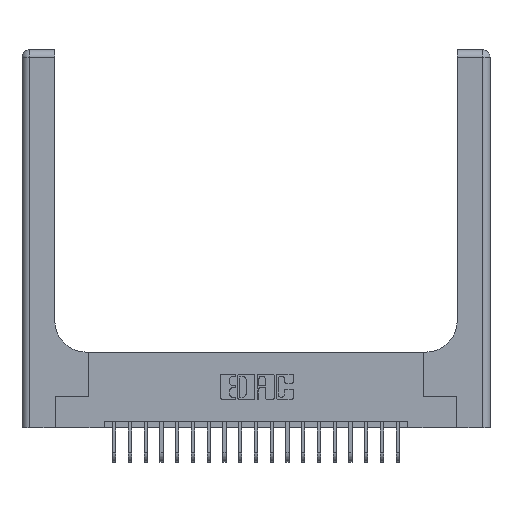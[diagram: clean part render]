
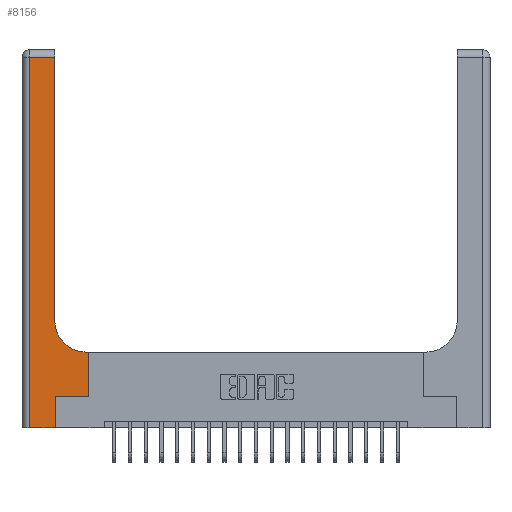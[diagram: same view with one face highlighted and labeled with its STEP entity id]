
A CAD part, top view. The second image highlights one B-rep face of the part: STEP entity #8156.
In plain terms, the highlighted planar face has unit normal (0, 0, 1).
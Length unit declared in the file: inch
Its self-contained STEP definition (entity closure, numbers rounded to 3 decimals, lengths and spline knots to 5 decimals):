
#72 = DIRECTION ( 'NONE',  ( -1., 0., 0. ) ) ;
#278 = ORIENTED_EDGE ( 'NONE', *, *, #3067, .T. ) ;
#315 = VERTEX_POINT ( 'NONE', #21766 ) ;
#575 = LINE ( 'NONE', #7647, #12299 ) ;
#623 = DIRECTION ( 'NONE',  ( -1., 0., 0. ) ) ;
#833 = ORIENTED_EDGE ( 'NONE', *, *, #17092, .T. ) ;
#1416 = EDGE_CURVE ( 'NONE', #14126, #315, #7775, .T. ) ;
#1889 = CARTESIAN_POINT ( 'NONE',  ( 0.528, 0.25, 0.37 ) ) ;
#1907 = EDGE_LOOP ( 'NONE', ( #4456, #3877, #278, #4391, #9613, #5532, #2901, #833, #2665 ) ) ;
#1970 = CARTESIAN_POINT ( 'NONE',  ( 0.528, 0.25, 0.37 ) ) ;
#2395 = CARTESIAN_POINT ( 'NONE',  ( 0.06, 0., 0.37 ) ) ;
#2665 = ORIENTED_EDGE ( 'NONE', *, *, #9471, .T. ) ;
#2901 = ORIENTED_EDGE ( 'NONE', *, *, #20682, .T. ) ;
#3067 = EDGE_CURVE ( 'NONE', #16271, #21588, #9029, .T. ) ;
#3318 = FACE_OUTER_BOUND ( 'NONE', #1907, .T. ) ;
#3342 = VERTEX_POINT ( 'NONE', #8316 ) ;
#3709 = DIRECTION ( 'NONE',  ( -1., 0., 0. ) ) ;
#3789 = CARTESIAN_POINT ( 'NONE',  ( 0., 2.94, 0.37 ) ) ;
#3877 = ORIENTED_EDGE ( 'NONE', *, *, #22731, .T. ) ;
#3880 = VECTOR ( 'NONE', #3709, 39.37008 ) ;
#3929 = CARTESIAN_POINT ( 'NONE',  ( 0.26, 0.6, 0.37 ) ) ;
#4391 = ORIENTED_EDGE ( 'NONE', *, *, #5251, .T. ) ;
#4456 = ORIENTED_EDGE ( 'NONE', *, *, #1416, .T. ) ;
#5196 = CIRCLE ( 'NONE', #21116, 0.25 ) ;
#5251 = EDGE_CURVE ( 'NONE', #21588, #14722, #5798, .T. ) ;
#5410 = VECTOR ( 'NONE', #12892, 39.37008 ) ;
#5532 = ORIENTED_EDGE ( 'NONE', *, *, #13686, .T. ) ;
#5798 = LINE ( 'NONE', #7873, #11797 ) ;
#6145 = DIRECTION ( 'NONE',  ( 1., 0., 0. ) ) ;
#7337 = VECTOR ( 'NONE', #14769, 39.37008 ) ;
#7448 = CARTESIAN_POINT ( 'NONE',  ( 0.528, 0.6, 0.37 ) ) ;
#7647 = CARTESIAN_POINT ( 'NONE',  ( 0.265, 0., 0.37 ) ) ;
#7775 = LINE ( 'NONE', #12660, #7337 ) ;
#7873 = CARTESIAN_POINT ( 'NONE',  ( 0., 0., 0.37 ) ) ;
#8156 = ADVANCED_FACE ( 'NONE', ( #3318 ), #12238, .F. ) ;
#8175 = AXIS2_PLACEMENT_3D ( 'NONE', #9310, #14686, #623 ) ;
#8316 = CARTESIAN_POINT ( 'NONE',  ( 0.51, 0.6, 0.37 ) ) ;
#8616 = CARTESIAN_POINT ( 'NONE',  ( 0.265, 0.25, 0.37 ) ) ;
#9029 = LINE ( 'NONE', #14277, #11999 ) ;
#9050 = VERTEX_POINT ( 'NONE', #19138 ) ;
#9310 = CARTESIAN_POINT ( 'NONE',  ( 0., 3., 0.37 ) ) ;
#9471 = EDGE_CURVE ( 'NONE', #3342, #14126, #5196, .T. ) ;
#9477 = VECTOR ( 'NONE', #72, 39.37008 ) ;
#9613 = ORIENTED_EDGE ( 'NONE', *, *, #11520, .T. ) ;
#10469 = DIRECTION ( 'NONE',  ( 1., 0., 0. ) ) ;
#11520 = EDGE_CURVE ( 'NONE', #14722, #9050, #575, .T. ) ;
#11797 = VECTOR ( 'NONE', #6145, 39.37008 ) ;
#11972 = CARTESIAN_POINT ( 'NONE',  ( 0.26, 0.85, 0.37 ) ) ;
#11999 = VECTOR ( 'NONE', #21327, 39.37008 ) ;
#12238 = PLANE ( 'NONE',  #8175 ) ;
#12299 = VECTOR ( 'NONE', #20290, 39.37008 ) ;
#12622 = VERTEX_POINT ( 'NONE', #7448 ) ;
#12660 = CARTESIAN_POINT ( 'NONE',  ( 0.26, 3., 0.37 ) ) ;
#12892 = DIRECTION ( 'NONE',  ( 0., 1., 0. ) ) ;
#13271 = CARTESIAN_POINT ( 'NONE',  ( 0.06, 2.94, 0.37 ) ) ;
#13686 = EDGE_CURVE ( 'NONE', #9050, #21127, #17445, .T. ) ;
#14126 = VERTEX_POINT ( 'NONE', #11972 ) ;
#14277 = CARTESIAN_POINT ( 'NONE',  ( 0.06, 3., 0.37 ) ) ;
#14387 = CARTESIAN_POINT ( 'NONE',  ( 0.265, 0., 0.37 ) ) ;
#14686 = DIRECTION ( 'NONE',  ( 0., 0., -1. ) ) ;
#14722 = VERTEX_POINT ( 'NONE', #14387 ) ;
#14769 = DIRECTION ( 'NONE',  ( 0., 1., 0. ) ) ;
#15997 = LINE ( 'NONE', #3789, #9477 ) ;
#16097 = VECTOR ( 'NONE', #10469, 39.37008 ) ;
#16271 = VERTEX_POINT ( 'NONE', #13271 ) ;
#17092 = EDGE_CURVE ( 'NONE', #12622, #3342, #19810, .T. ) ;
#17445 = LINE ( 'NONE', #8616, #16097 ) ;
#17568 = DIRECTION ( 'NONE',  ( 0., 0., -1. ) ) ;
#19138 = CARTESIAN_POINT ( 'NONE',  ( 0.265, 0.25, 0.37 ) ) ;
#19810 = LINE ( 'NONE', #3929, #3880 ) ;
#20290 = DIRECTION ( 'NONE',  ( 0., 1., 0. ) ) ;
#20682 = EDGE_CURVE ( 'NONE', #21127, #12622, #21569, .T. ) ;
#21116 = AXIS2_PLACEMENT_3D ( 'NONE', #21274, #17568, #22896 ) ;
#21127 = VERTEX_POINT ( 'NONE', #1970 ) ;
#21274 = CARTESIAN_POINT ( 'NONE',  ( 0.51, 0.85, 0.37 ) ) ;
#21327 = DIRECTION ( 'NONE',  ( 0., -1., 0. ) ) ;
#21569 = LINE ( 'NONE', #1889, #5410 ) ;
#21588 = VERTEX_POINT ( 'NONE', #2395 ) ;
#21766 = CARTESIAN_POINT ( 'NONE',  ( 0.26, 2.94, 0.37 ) ) ;
#22731 = EDGE_CURVE ( 'NONE', #315, #16271, #15997, .T. ) ;
#22896 = DIRECTION ( 'NONE',  ( 1., 0., 0. ) ) ;
